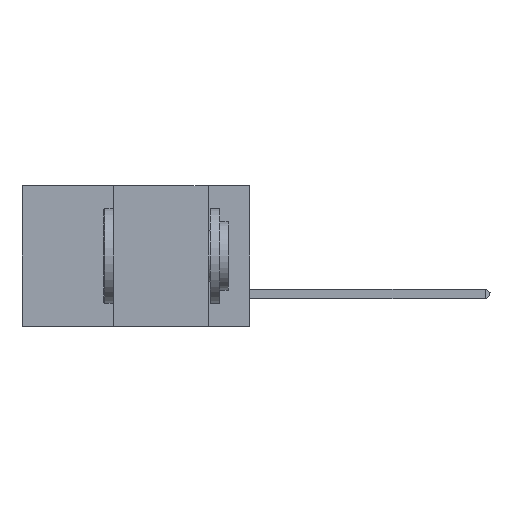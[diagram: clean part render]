
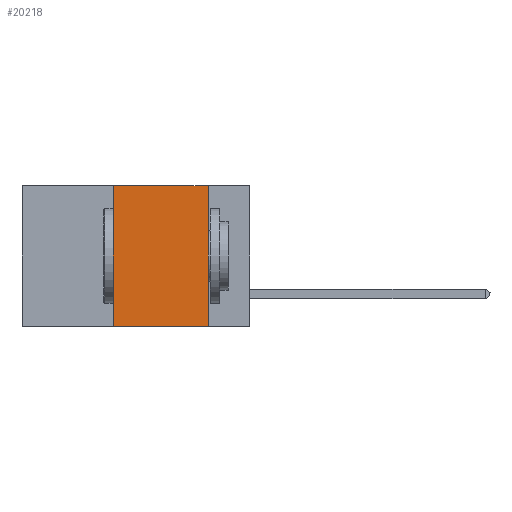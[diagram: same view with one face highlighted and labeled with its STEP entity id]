
A CAD part, left-side view. The second image highlights one B-rep face of the part: STEP entity #20218.
In plain terms, the highlighted planar face has unit normal (-1, 0, 0).
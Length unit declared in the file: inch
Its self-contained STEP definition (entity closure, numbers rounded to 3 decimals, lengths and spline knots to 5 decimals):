
#397 = LINE ( 'NONE', #42861, #33505 ) ;
#2889 = VERTEX_POINT ( 'NONE', #27240 ) ;
#2997 = EDGE_CURVE ( 'NONE', #23021, #2889, #20020, .T. ) ;
#3042 = FACE_OUTER_BOUND ( 'NONE', #32768, .T. ) ;
#6868 = VECTOR ( 'NONE', #42936, 39.37008 ) ;
#7190 = EDGE_CURVE ( 'NONE', #40832, #23021, #38840, .T. ) ;
#8065 = CARTESIAN_POINT ( 'NONE',  ( 0., 0.36, 0. ) ) ;
#8425 = CARTESIAN_POINT ( 'NONE',  ( 0., 0.6, -0.37 ) ) ;
#9016 = CARTESIAN_POINT ( 'NONE',  ( 0., 0.6, 0. ) ) ;
#11867 = VERTEX_POINT ( 'NONE', #13019 ) ;
#12665 = PLANE ( 'NONE',  #30905 ) ;
#13019 = CARTESIAN_POINT ( 'NONE',  ( 0., 0.36, -0.37 ) ) ;
#13819 = CARTESIAN_POINT ( 'NONE',  ( 0., 0.6, 0. ) ) ;
#14061 = EDGE_CURVE ( 'NONE', #11867, #40832, #397, .T. ) ;
#16761 = ORIENTED_EDGE ( 'NONE', *, *, #7190, .F. ) ;
#17821 = ORIENTED_EDGE ( 'NONE', *, *, #32323, .T. ) ;
#20020 = LINE ( 'NONE', #21465, #40365 ) ;
#20218 = ADVANCED_FACE ( 'NONE', ( #3042 ), #12665, .F. ) ;
#20695 = VECTOR ( 'NONE', #41256, 39.37008 ) ;
#21465 = CARTESIAN_POINT ( 'NONE',  ( 0., 0.11, 0. ) ) ;
#23021 = VERTEX_POINT ( 'NONE', #39180 ) ;
#27240 = CARTESIAN_POINT ( 'NONE',  ( 0., 0.11, -0.37 ) ) ;
#30905 = AXIS2_PLACEMENT_3D ( 'NONE', #13819, #41089, #40825 ) ;
#32323 = EDGE_CURVE ( 'NONE', #11867, #2889, #39973, .T. ) ;
#32768 = EDGE_LOOP ( 'NONE', ( #35325, #16761, #37407, #17821 ) ) ;
#33505 = VECTOR ( 'NONE', #36127, 39.37008 ) ;
#35325 = ORIENTED_EDGE ( 'NONE', *, *, #2997, .F. ) ;
#36111 = DIRECTION ( 'NONE',  ( 0., 0., -1. ) ) ;
#36127 = DIRECTION ( 'NONE',  ( 0., 0., 1. ) ) ;
#37407 = ORIENTED_EDGE ( 'NONE', *, *, #14061, .F. ) ;
#38840 = LINE ( 'NONE', #9016, #20695 ) ;
#39180 = CARTESIAN_POINT ( 'NONE',  ( 0., 0.11, 0. ) ) ;
#39973 = LINE ( 'NONE', #8425, #6868 ) ;
#40365 = VECTOR ( 'NONE', #36111, 39.37008 ) ;
#40825 = DIRECTION ( 'NONE',  ( 0., 0., -1. ) ) ;
#40832 = VERTEX_POINT ( 'NONE', #8065 ) ;
#41089 = DIRECTION ( 'NONE',  ( 1., 0., 0. ) ) ;
#41256 = DIRECTION ( 'NONE',  ( 0., -1., 0. ) ) ;
#42861 = CARTESIAN_POINT ( 'NONE',  ( 0., 0.36, 0. ) ) ;
#42936 = DIRECTION ( 'NONE',  ( 0., -1., 0. ) ) ;
